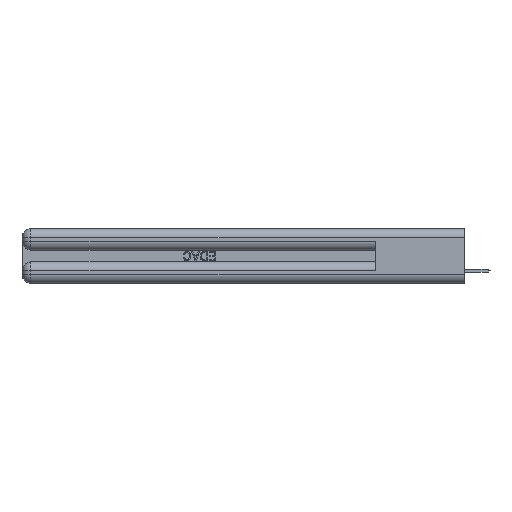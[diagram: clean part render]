
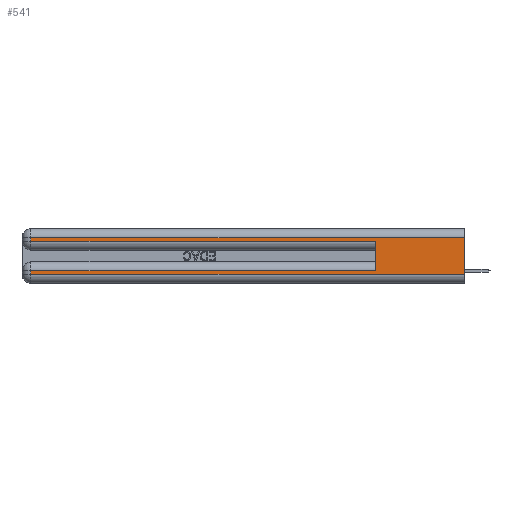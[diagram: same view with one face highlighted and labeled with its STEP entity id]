
A CAD part, left-side view. The second image highlights one B-rep face of the part: STEP entity #541.
In plain terms, the highlighted planar face has unit normal (-1, 0, 0).
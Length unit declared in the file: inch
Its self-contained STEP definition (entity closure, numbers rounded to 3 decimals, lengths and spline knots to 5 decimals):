
#264 = VERTEX_POINT ( 'NONE', #29218 ) ;
#541 = ADVANCED_FACE ( 'NONE', ( #16858 ), #1884, .F. ) ;
#591 = CARTESIAN_POINT ( 'NONE',  ( 0., 0., 0.085 ) ) ;
#1287 = DIRECTION ( 'NONE',  ( 0., -1., 0. ) ) ;
#1884 = PLANE ( 'NONE',  #2970 ) ;
#2843 = ORIENTED_EDGE ( 'NONE', *, *, #31657, .T. ) ;
#2902 = VECTOR ( 'NONE', #1287, 39.37008 ) ;
#2970 = AXIS2_PLACEMENT_3D ( 'NONE', #33572, #19062, #29629 ) ;
#3194 = LINE ( 'NONE', #44457, #39403 ) ;
#3326 = CARTESIAN_POINT ( 'NONE',  ( 0., 0.6, 0.145 ) ) ;
#4528 = ORIENTED_EDGE ( 'NONE', *, *, #43236, .T. ) ;
#5575 = VECTOR ( 'NONE', #24545, 39.37008 ) ;
#6213 = VERTEX_POINT ( 'NONE', #33676 ) ;
#7357 = CARTESIAN_POINT ( 'NONE',  ( 0., 0., 0.06 ) ) ;
#7944 = LINE ( 'NONE', #25576, #14526 ) ;
#8124 = ORIENTED_EDGE ( 'NONE', *, *, #24317, .T. ) ;
#9234 = LINE ( 'NONE', #19786, #40535 ) ;
#10363 = CARTESIAN_POINT ( 'NONE',  ( 0., 2.94, 0.285 ) ) ;
#10448 = VERTEX_POINT ( 'NONE', #7357 ) ;
#10639 = VECTOR ( 'NONE', #36169, 39.37008 ) ;
#12179 = CARTESIAN_POINT ( 'NONE',  ( 0., 2.94, 0.37 ) ) ;
#12847 = LINE ( 'NONE', #29920, #31069 ) ;
#13806 = VERTEX_POINT ( 'NONE', #10363 ) ;
#14526 = VECTOR ( 'NONE', #42758, 39.37008 ) ;
#14878 = CARTESIAN_POINT ( 'NONE',  ( 0., 0.6, 0.285 ) ) ;
#15611 = VERTEX_POINT ( 'NONE', #43914 ) ;
#16858 = FACE_OUTER_BOUND ( 'NONE', #41223, .T. ) ;
#19062 = DIRECTION ( 'NONE',  ( 1., 0., 0. ) ) ;
#19145 = EDGE_CURVE ( 'NONE', #28363, #10448, #3194, .T. ) ;
#19183 = VECTOR ( 'NONE', #29919, 39.37008 ) ;
#19786 = CARTESIAN_POINT ( 'NONE',  ( 0., 0., 0.06 ) ) ;
#22496 = DIRECTION ( 'NONE',  ( 0., 0., -1. ) ) ;
#22918 = CARTESIAN_POINT ( 'NONE',  ( 0., 0., 0.31 ) ) ;
#23066 = LINE ( 'NONE', #591, #19183 ) ;
#23760 = LINE ( 'NONE', #3326, #5575 ) ;
#23903 = DIRECTION ( 'NONE',  ( 0., 0., -1. ) ) ;
#24317 = EDGE_CURVE ( 'NONE', #28363, #28401, #7944, .T. ) ;
#24545 = DIRECTION ( 'NONE',  ( 0., 0., 1. ) ) ;
#24952 = EDGE_CURVE ( 'NONE', #28401, #13806, #32633, .T. ) ;
#25576 = CARTESIAN_POINT ( 'NONE',  ( 0., 0., 0.31 ) ) ;
#26369 = VERTEX_POINT ( 'NONE', #14878 ) ;
#28363 = VERTEX_POINT ( 'NONE', #22918 ) ;
#28401 = VERTEX_POINT ( 'NONE', #29383 ) ;
#29218 = CARTESIAN_POINT ( 'NONE',  ( 0., 2.94, 0.06 ) ) ;
#29383 = CARTESIAN_POINT ( 'NONE',  ( 0., 2.94, 0.31 ) ) ;
#29629 = DIRECTION ( 'NONE',  ( 0., 0., -1. ) ) ;
#29758 = ORIENTED_EDGE ( 'NONE', *, *, #19145, .F. ) ;
#29815 = ORIENTED_EDGE ( 'NONE', *, *, #42057, .T. ) ;
#29919 = DIRECTION ( 'NONE',  ( 0., 1., 0. ) ) ;
#29920 = CARTESIAN_POINT ( 'NONE',  ( 0., 2.94, 0.37 ) ) ;
#29960 = CARTESIAN_POINT ( 'NONE',  ( 0., 0., 0.285 ) ) ;
#31069 = VECTOR ( 'NONE', #22496, 39.37008 ) ;
#31657 = EDGE_CURVE ( 'NONE', #15611, #264, #12847, .T. ) ;
#32633 = LINE ( 'NONE', #12179, #10639 ) ;
#33093 = EDGE_CURVE ( 'NONE', #6213, #26369, #23760, .T. ) ;
#33572 = CARTESIAN_POINT ( 'NONE',  ( 0., 0., 0.37 ) ) ;
#33676 = CARTESIAN_POINT ( 'NONE',  ( 0., 0.6, 0.085 ) ) ;
#34220 = ORIENTED_EDGE ( 'NONE', *, *, #24952, .T. ) ;
#36169 = DIRECTION ( 'NONE',  ( 0., 0., -1. ) ) ;
#36848 = DIRECTION ( 'NONE',  ( 0., -1., 0. ) ) ;
#39403 = VECTOR ( 'NONE', #23903, 39.37008 ) ;
#39986 = EDGE_CURVE ( 'NONE', #13806, #26369, #43543, .T. ) ;
#40535 = VECTOR ( 'NONE', #36848, 39.37008 ) ;
#41223 = EDGE_LOOP ( 'NONE', ( #29758, #8124, #34220, #41702, #42582, #29815, #2843, #4528 ) ) ;
#41702 = ORIENTED_EDGE ( 'NONE', *, *, #39986, .T. ) ;
#42057 = EDGE_CURVE ( 'NONE', #6213, #15611, #23066, .T. ) ;
#42582 = ORIENTED_EDGE ( 'NONE', *, *, #33093, .F. ) ;
#42758 = DIRECTION ( 'NONE',  ( 0., 1., 0. ) ) ;
#43236 = EDGE_CURVE ( 'NONE', #264, #10448, #9234, .T. ) ;
#43543 = LINE ( 'NONE', #29960, #2902 ) ;
#43914 = CARTESIAN_POINT ( 'NONE',  ( 0., 2.94, 0.085 ) ) ;
#44457 = CARTESIAN_POINT ( 'NONE',  ( 0., 0., 0.37 ) ) ;
